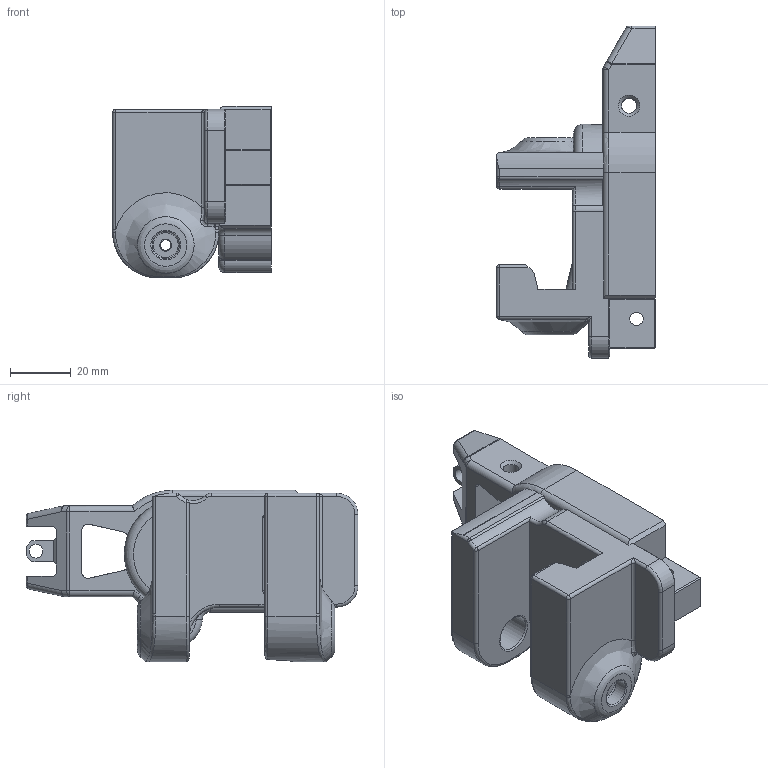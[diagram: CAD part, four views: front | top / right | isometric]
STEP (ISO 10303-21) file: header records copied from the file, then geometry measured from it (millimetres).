
FILE_DESCRIPTION (( 'STEP AP203' ), '1' );
FILE_NAME ('MOD9_endcap_IS.STEP', '2020-08-28T04:23:14', ( '' ), ( '' ), 'SwSTEP 2.0', 'SolidWorks 2016', '' );
FILE_SCHEMA (( 'CONFIG_CONTROL_DESIGN' ));
Length unit declared in the file: millimetre
Products named in the file (1): MOD9_endcap_IS
Bounding box: 52.33 x 109.4 x 56.54 mm (x, y, z)
Volume: 111379.2 mm3; surface area: 26914.3 mm2
Topology: 1 solids, 1 shells, 243 faces, 621 edges, 378 vertices
Faces by surface type: plane 90, cylinder 80, torus 31, bspline 22, cone 11, sphere 9
Full cylindrical faces by diameter (mm): 3.4 x1, 4 x1, 4.4 x1, 4.5 x1, 5 x2, 9 x1, 12 x1, 23 x1
Entity records: 8463 total; most frequent: CARTESIAN_POINT 2872, ORIENTED_EDGE 1174, DIRECTION 1080, EDGE_CURVE 587, AXIS2_PLACEMENT_3D 396, VERTEX_POINT 371, LINE 288, VECTOR 288
